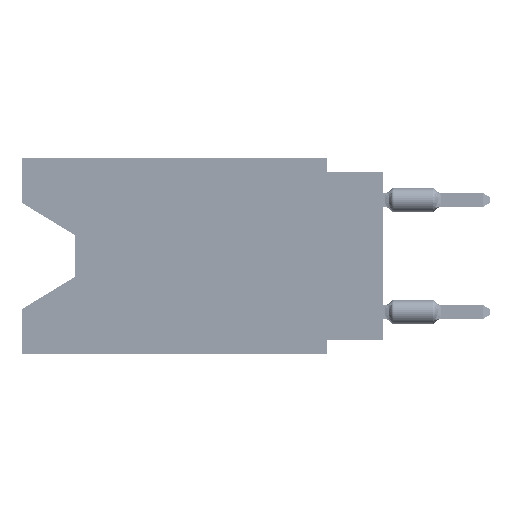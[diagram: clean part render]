
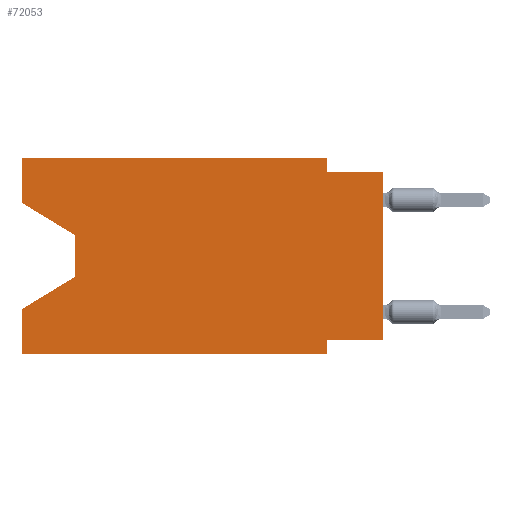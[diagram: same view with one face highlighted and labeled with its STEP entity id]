
A CAD part, left-side view. The second image highlights one B-rep face of the part: STEP entity #72053.
In plain terms, the highlighted planar face has unit normal (-1, 0, 0).
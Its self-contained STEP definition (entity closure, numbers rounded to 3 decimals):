
#233 = VERTEX_POINT ( 'NONE', #31722 ) ;
#427 = DIRECTION ( 'NONE',  ( 0., -0.855, -0.519 ) ) ;
#1084 = LINE ( 'NONE', #28508, #20617 ) ;
#1351 = ORIENTED_EDGE ( 'NONE', *, *, #12078, .F. ) ;
#3551 = CARTESIAN_POINT ( 'NONE',  ( 0., 16.383, 0. ) ) ;
#5913 = LINE ( 'NONE', #44339, #63989 ) ;
#6521 = VECTOR ( 'NONE', #51283, 1000. ) ;
#7363 = VERTEX_POINT ( 'NONE', #64130 ) ;
#7411 = CARTESIAN_POINT ( 'NONE',  ( 0., 2.54, -8.89 ) ) ;
#7762 = CARTESIAN_POINT ( 'NONE',  ( 0., 2.54, 0. ) ) ;
#9048 = PLANE ( 'NONE',  #66903 ) ;
#9766 = DIRECTION ( 'NONE',  ( 0., 0., -1. ) ) ;
#10822 = EDGE_CURVE ( 'NONE', #19970, #53560, #52377, .T. ) ;
#11458 = DIRECTION ( 'NONE',  ( 0., 0., 1. ) ) ;
#11915 = CARTESIAN_POINT ( 'NONE',  ( 0., 13.97, -3.505 ) ) ;
#12078 = EDGE_CURVE ( 'NONE', #53560, #66816, #69216, .T. ) ;
#12853 = VECTOR ( 'NONE', #54018, 1000. ) ;
#13648 = EDGE_CURVE ( 'NONE', #28565, #233, #34392, .T. ) ;
#14072 = VECTOR ( 'NONE', #14493, 1000. ) ;
#14493 = DIRECTION ( 'NONE',  ( 0., 0., 1. ) ) ;
#14677 = CARTESIAN_POINT ( 'NONE',  ( 0., 0., -8.255 ) ) ;
#14884 = ORIENTED_EDGE ( 'NONE', *, *, #67740, .F. ) ;
#15317 = CARTESIAN_POINT ( 'NONE',  ( 0., 16.383, -2.038 ) ) ;
#15613 = CARTESIAN_POINT ( 'NONE',  ( 0., 16.383, 0. ) ) ;
#15615 = VERTEX_POINT ( 'NONE', #41945 ) ;
#15895 = EDGE_CURVE ( 'NONE', #36695, #62228, #28013, .T. ) ;
#16027 = CARTESIAN_POINT ( 'NONE',  ( 0., 13.97, -5.385 ) ) ;
#16075 = CARTESIAN_POINT ( 'NONE',  ( 0., 16.383, -8.89 ) ) ;
#19442 = VECTOR ( 'NONE', #32792, 1000. ) ;
#19808 = DIRECTION ( 'NONE',  ( 0., 1., 0. ) ) ;
#19970 = VERTEX_POINT ( 'NONE', #58481 ) ;
#20617 = VECTOR ( 'NONE', #23029, 1000. ) ;
#20743 = FACE_OUTER_BOUND ( 'NONE', #61594, .T. ) ;
#21103 = DIRECTION ( 'NONE',  ( 1., 0., 0. ) ) ;
#22463 = CARTESIAN_POINT ( 'NONE',  ( 0., 2.54, 0. ) ) ;
#22773 = CARTESIAN_POINT ( 'NONE',  ( 0., 2.54, -8.255 ) ) ;
#23029 = DIRECTION ( 'NONE',  ( 0., 0.855, -0.519 ) ) ;
#24936 = LINE ( 'NONE', #7762, #6521 ) ;
#28013 = LINE ( 'NONE', #50321, #70857 ) ;
#28319 = ORIENTED_EDGE ( 'NONE', *, *, #59627, .T. ) ;
#28508 = CARTESIAN_POINT ( 'NONE',  ( 0., 13.97, -5.385 ) ) ;
#28565 = VERTEX_POINT ( 'NONE', #30328 ) ;
#29712 = DIRECTION ( 'NONE',  ( 0., 0., -1. ) ) ;
#30328 = CARTESIAN_POINT ( 'NONE',  ( 0., 2.54, -0.635 ) ) ;
#31690 = ORIENTED_EDGE ( 'NONE', *, *, #10822, .F. ) ;
#31722 = CARTESIAN_POINT ( 'NONE',  ( 0., 0., -0.635 ) ) ;
#32792 = DIRECTION ( 'NONE',  ( 0., -1., 0. ) ) ;
#33756 = CARTESIAN_POINT ( 'NONE',  ( 0., 0., 0. ) ) ;
#34209 = EDGE_CURVE ( 'NONE', #57995, #28565, #24936, .T. ) ;
#34392 = LINE ( 'NONE', #41705, #34566 ) ;
#34566 = VECTOR ( 'NONE', #45742, 1000. ) ;
#36227 = ORIENTED_EDGE ( 'NONE', *, *, #53040, .F. ) ;
#36695 = VERTEX_POINT ( 'NONE', #11915 ) ;
#37098 = VECTOR ( 'NONE', #29712, 1000. ) ;
#37524 = CARTESIAN_POINT ( 'NONE',  ( 0., 16.383, 0. ) ) ;
#37540 = ORIENTED_EDGE ( 'NONE', *, *, #37656, .F. ) ;
#37656 = EDGE_CURVE ( 'NONE', #68590, #72297, #53654, .T. ) ;
#38576 = VECTOR ( 'NONE', #43871, 1000. ) ;
#41705 = CARTESIAN_POINT ( 'NONE',  ( 0., 0., -0.635 ) ) ;
#41945 = CARTESIAN_POINT ( 'NONE',  ( 0., 16.383, -6.852 ) ) ;
#42509 = ORIENTED_EDGE ( 'NONE', *, *, #15895, .T. ) ;
#43871 = DIRECTION ( 'NONE',  ( 0., -1., 0. ) ) ;
#44339 = CARTESIAN_POINT ( 'NONE',  ( 0., 16.383, -2.038 ) ) ;
#45311 = EDGE_CURVE ( 'NONE', #7363, #66816, #54477, .T. ) ;
#45589 = ORIENTED_EDGE ( 'NONE', *, *, #13648, .F. ) ;
#45742 = DIRECTION ( 'NONE',  ( 0., -1., 0. ) ) ;
#46556 = EDGE_CURVE ( 'NONE', #62228, #15615, #1084, .T. ) ;
#47971 = ORIENTED_EDGE ( 'NONE', *, *, #34209, .F. ) ;
#50321 = CARTESIAN_POINT ( 'NONE',  ( 0., 13.97, -3.505 ) ) ;
#51283 = DIRECTION ( 'NONE',  ( 0., 0., -1. ) ) ;
#52377 = LINE ( 'NONE', #14677, #72031 ) ;
#53040 = EDGE_CURVE ( 'NONE', #72297, #57995, #66449, .T. ) ;
#53560 = VERTEX_POINT ( 'NONE', #22773 ) ;
#53654 = LINE ( 'NONE', #3551, #12853 ) ;
#53989 = LINE ( 'NONE', #37524, #14072 ) ;
#54018 = DIRECTION ( 'NONE',  ( 0., 0., 1. ) ) ;
#54477 = LINE ( 'NONE', #16075, #38576 ) ;
#55776 = ORIENTED_EDGE ( 'NONE', *, *, #45311, .T. ) ;
#56510 = DIRECTION ( 'NONE',  ( 0., 0., -1. ) ) ;
#57995 = VERTEX_POINT ( 'NONE', #22463 ) ;
#58481 = CARTESIAN_POINT ( 'NONE',  ( 0., 0., -8.255 ) ) ;
#59288 = CARTESIAN_POINT ( 'NONE',  ( 0., 2.54, -8.89 ) ) ;
#59627 = EDGE_CURVE ( 'NONE', #68590, #36695, #5913, .T. ) ;
#61237 = ORIENTED_EDGE ( 'NONE', *, *, #46556, .T. ) ;
#61571 = LINE ( 'NONE', #33756, #71331 ) ;
#61594 = EDGE_LOOP ( 'NONE', ( #28319, #42509, #61237, #14884, #55776, #1351, #31690, #68266, #45589, #47971, #36227, #37540 ) ) ;
#62228 = VERTEX_POINT ( 'NONE', #16027 ) ;
#63989 = VECTOR ( 'NONE', #427, 1000. ) ;
#64130 = CARTESIAN_POINT ( 'NONE',  ( 0., 16.383, -8.89 ) ) ;
#64197 = CARTESIAN_POINT ( 'NONE',  ( 0., 16.383, 0. ) ) ;
#66449 = LINE ( 'NONE', #71576, #19442 ) ;
#66816 = VERTEX_POINT ( 'NONE', #59288 ) ;
#66903 = AXIS2_PLACEMENT_3D ( 'NONE', #15613, #21103, #9766 ) ;
#67740 = EDGE_CURVE ( 'NONE', #7363, #15615, #53989, .T. ) ;
#68266 = ORIENTED_EDGE ( 'NONE', *, *, #69733, .T. ) ;
#68590 = VERTEX_POINT ( 'NONE', #15317 ) ;
#69216 = LINE ( 'NONE', #7411, #37098 ) ;
#69733 = EDGE_CURVE ( 'NONE', #19970, #233, #61571, .T. ) ;
#70857 = VECTOR ( 'NONE', #56510, 1000. ) ;
#71331 = VECTOR ( 'NONE', #11458, 1000. ) ;
#71576 = CARTESIAN_POINT ( 'NONE',  ( 0., 16.383, 0. ) ) ;
#72031 = VECTOR ( 'NONE', #19808, 1000. ) ;
#72053 = ADVANCED_FACE ( 'NONE', ( #20743 ), #9048, .F. ) ;
#72297 = VERTEX_POINT ( 'NONE', #64197 ) ;
